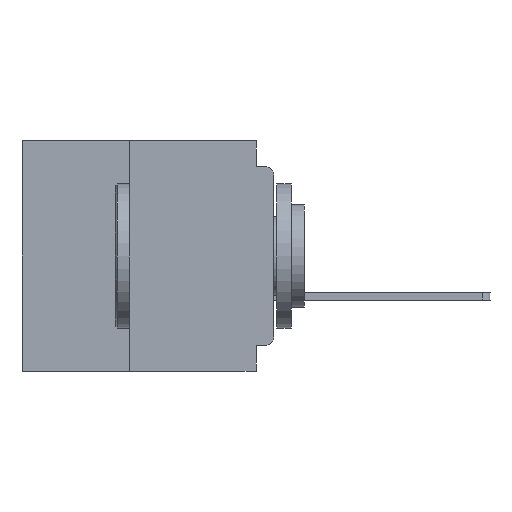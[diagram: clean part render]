
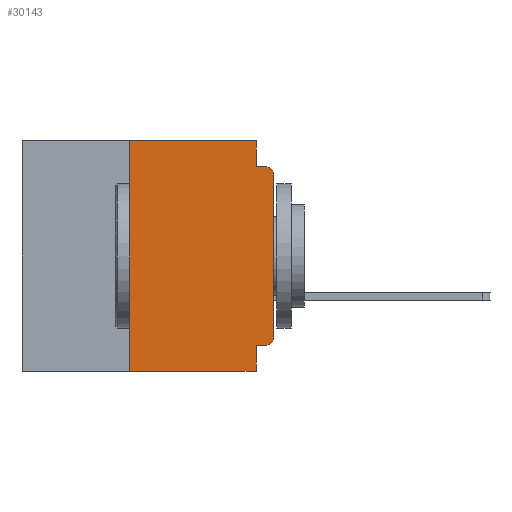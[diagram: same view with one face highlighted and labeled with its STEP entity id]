
A CAD part, left-side view. The second image highlights one B-rep face of the part: STEP entity #30143.
In plain terms, the highlighted planar face has unit normal (-1, 0, 0).
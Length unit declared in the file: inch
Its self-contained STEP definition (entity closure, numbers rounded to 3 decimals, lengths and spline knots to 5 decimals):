
#389 = CARTESIAN_POINT ( 'NONE',  ( 0., 0.031, 0. ) ) ;
#826 = DIRECTION ( 'NONE',  ( 0., -1., 0. ) ) ;
#2002 = ORIENTED_EDGE ( 'NONE', *, *, #54405, .T. ) ;
#2270 = EDGE_LOOP ( 'NONE', ( #2002, #2565, #29915, #23760, #65830, #61108, #43281, #2737, #29984, #25170 ) ) ;
#2565 = ORIENTED_EDGE ( 'NONE', *, *, #37634, .T. ) ;
#2677 = CARTESIAN_POINT ( 'NONE',  ( 0., 0.031, -0.4 ) ) ;
#2696 = LINE ( 'NONE', #7619, #18513 ) ;
#2737 = ORIENTED_EDGE ( 'NONE', *, *, #36272, .F. ) ;
#2819 = VERTEX_POINT ( 'NONE', #44986 ) ;
#2949 = EDGE_CURVE ( 'NONE', #61778, #9021, #9239, .T. ) ;
#4203 = DIRECTION ( 'NONE',  ( 0., 0., 1. ) ) ;
#4637 = AXIS2_PLACEMENT_3D ( 'NONE', #25175, #61952, #30480 ) ;
#5940 = VERTEX_POINT ( 'NONE', #41891 ) ;
#6702 = CARTESIAN_POINT ( 'NONE',  ( 0., 0., -0.355 ) ) ;
#7619 = CARTESIAN_POINT ( 'NONE',  ( 0., 0.031, -0.4 ) ) ;
#9021 = VERTEX_POINT ( 'NONE', #34207 ) ;
#9239 = LINE ( 'NONE', #35125, #63490 ) ;
#9387 = CIRCLE ( 'NONE', #26247, 0.015 ) ;
#10744 = PLANE ( 'NONE',  #58073 ) ;
#12050 = DIRECTION ( 'NONE',  ( 0., 1., 0. ) ) ;
#12445 = EDGE_CURVE ( 'NONE', #2819, #53600, #42677, .T. ) ;
#13233 = LINE ( 'NONE', #27423, #23925 ) ;
#14275 = CARTESIAN_POINT ( 'NONE',  ( 0., 0., -0.06 ) ) ;
#15179 = EDGE_CURVE ( 'NONE', #5940, #39419, #13233, .T. ) ;
#17233 = VECTOR ( 'NONE', #12050, 39.37008 ) ;
#18513 = VECTOR ( 'NONE', #39080, 39.37008 ) ;
#19841 = DIRECTION ( 'NONE',  ( 0., -1., 0. ) ) ;
#23090 = VERTEX_POINT ( 'NONE', #14275 ) ;
#23760 = ORIENTED_EDGE ( 'NONE', *, *, #23935, .F. ) ;
#23925 = VECTOR ( 'NONE', #826, 39.37008 ) ;
#23935 = EDGE_CURVE ( 'NONE', #39419, #61778, #67014, .T. ) ;
#25005 = DIRECTION ( 'NONE',  ( 0., -1., 0. ) ) ;
#25170 = ORIENTED_EDGE ( 'NONE', *, *, #52729, .T. ) ;
#25175 = CARTESIAN_POINT ( 'NONE',  ( 0., 0.015, -0.06 ) ) ;
#26247 = AXIS2_PLACEMENT_3D ( 'NONE', #62558, #31094, #67830 ) ;
#26448 = CARTESIAN_POINT ( 'NONE',  ( 0., 0.015, -0.355 ) ) ;
#26591 = CARTESIAN_POINT ( 'NONE',  ( 0., 0.437, 0. ) ) ;
#26798 = CARTESIAN_POINT ( 'NONE',  ( 0., 0.031, 0. ) ) ;
#26817 = CARTESIAN_POINT ( 'NONE',  ( 0., 0.031, -0.045 ) ) ;
#27423 = CARTESIAN_POINT ( 'NONE',  ( 0., 0.437, 0. ) ) ;
#28736 = VECTOR ( 'NONE', #19841, 39.37008 ) ;
#29915 = ORIENTED_EDGE ( 'NONE', *, *, #2949, .F. ) ;
#29984 = ORIENTED_EDGE ( 'NONE', *, *, #45601, .F. ) ;
#30143 = ADVANCED_FACE ( 'NONE', ( #51323 ), #10744, .F. ) ;
#30480 = DIRECTION ( 'NONE',  ( 0., 0., -1. ) ) ;
#31094 = DIRECTION ( 'NONE',  ( -1., 0., 0. ) ) ;
#31885 = DIRECTION ( 'NONE',  ( 0., 0., -1. ) ) ;
#33780 = CARTESIAN_POINT ( 'NONE',  ( 0., 0., -0.34 ) ) ;
#34207 = CARTESIAN_POINT ( 'NONE',  ( 0., 0.015, -0.045 ) ) ;
#35125 = CARTESIAN_POINT ( 'NONE',  ( 0., 0., -0.045 ) ) ;
#35775 = CARTESIAN_POINT ( 'NONE',  ( 0., 0., 0. ) ) ;
#36272 = EDGE_CURVE ( 'NONE', #45412, #53600, #2696, .T. ) ;
#36868 = VERTEX_POINT ( 'NONE', #33780 ) ;
#37634 = EDGE_CURVE ( 'NONE', #23090, #9021, #58111, .T. ) ;
#38273 = LINE ( 'NONE', #47232, #64613 ) ;
#39080 = DIRECTION ( 'NONE',  ( 0., 0., -1. ) ) ;
#39419 = VERTEX_POINT ( 'NONE', #26798 ) ;
#41891 = CARTESIAN_POINT ( 'NONE',  ( 0., 0.25, 0. ) ) ;
#42677 = LINE ( 'NONE', #51266, #28736 ) ;
#43281 = ORIENTED_EDGE ( 'NONE', *, *, #12445, .T. ) ;
#43431 = LINE ( 'NONE', #6702, #17233 ) ;
#44885 = LINE ( 'NONE', #35775, #58902 ) ;
#44986 = CARTESIAN_POINT ( 'NONE',  ( 0., 0.25, -0.4 ) ) ;
#45412 = VERTEX_POINT ( 'NONE', #57580 ) ;
#45601 = EDGE_CURVE ( 'NONE', #55679, #45412, #43431, .T. ) ;
#47232 = CARTESIAN_POINT ( 'NONE',  ( 0., 0.25, -0.4 ) ) ;
#51266 = CARTESIAN_POINT ( 'NONE',  ( 0., 0.437, -0.4 ) ) ;
#51323 = FACE_OUTER_BOUND ( 'NONE', #2270, .T. ) ;
#52566 = DIRECTION ( 'NONE',  ( 0., 0., 1. ) ) ;
#52729 = EDGE_CURVE ( 'NONE', #55679, #36868, #9387, .T. ) ;
#53600 = VERTEX_POINT ( 'NONE', #2677 ) ;
#54405 = EDGE_CURVE ( 'NONE', #36868, #23090, #44885, .T. ) ;
#54529 = EDGE_CURVE ( 'NONE', #2819, #5940, #38273, .T. ) ;
#55679 = VERTEX_POINT ( 'NONE', #26448 ) ;
#57580 = CARTESIAN_POINT ( 'NONE',  ( 0., 0.031, -0.355 ) ) ;
#58073 = AXIS2_PLACEMENT_3D ( 'NONE', #26591, #63358, #31885 ) ;
#58111 = CIRCLE ( 'NONE', #4637, 0.015 ) ;
#58252 = DIRECTION ( 'NONE',  ( 0., 0., -1. ) ) ;
#58902 = VECTOR ( 'NONE', #4203, 39.37008 ) ;
#61108 = ORIENTED_EDGE ( 'NONE', *, *, #54529, .F. ) ;
#61778 = VERTEX_POINT ( 'NONE', #26817 ) ;
#61952 = DIRECTION ( 'NONE',  ( -1., 0., 0. ) ) ;
#62558 = CARTESIAN_POINT ( 'NONE',  ( 0., 0.015, -0.34 ) ) ;
#63358 = DIRECTION ( 'NONE',  ( 1., 0., 0. ) ) ;
#63490 = VECTOR ( 'NONE', #25005, 39.37008 ) ;
#63727 = VECTOR ( 'NONE', #58252, 39.37008 ) ;
#64613 = VECTOR ( 'NONE', #52566, 39.37008 ) ;
#65830 = ORIENTED_EDGE ( 'NONE', *, *, #15179, .F. ) ;
#67014 = LINE ( 'NONE', #389, #63727 ) ;
#67830 = DIRECTION ( 'NONE',  ( 0., 0., -1. ) ) ;
